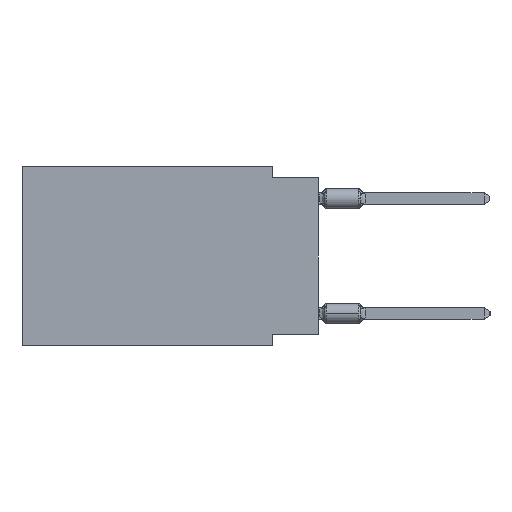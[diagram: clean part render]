
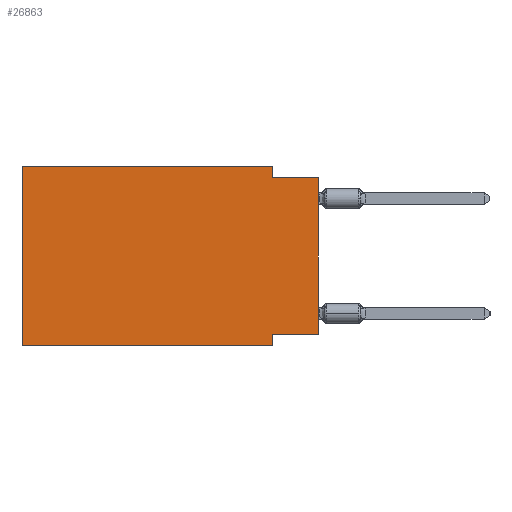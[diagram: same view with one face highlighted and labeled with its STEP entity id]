
A CAD part, left-side view. The second image highlights one B-rep face of the part: STEP entity #26863.
In plain terms, the highlighted planar face has unit normal (-1, 0, 0).
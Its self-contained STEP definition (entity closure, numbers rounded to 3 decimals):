
#726 = DIRECTION ( 'NONE',  ( 1., 0., 0. ) ) ;
#761 = DIRECTION ( 'NONE',  ( 0., -1., 0. ) ) ;
#893 = CARTESIAN_POINT ( 'NONE',  ( 0., 0., -0.635 ) ) ;
#2442 = CARTESIAN_POINT ( 'NONE',  ( 0., 16.383, 0. ) ) ;
#2664 = EDGE_CURVE ( 'NONE', #21408, #15337, #25384, .T. ) ;
#2811 = VECTOR ( 'NONE', #15231, 1000. ) ;
#2906 = CARTESIAN_POINT ( 'NONE',  ( 0., 16.383, 0. ) ) ;
#3596 = CARTESIAN_POINT ( 'NONE',  ( 0., 16.383, 0. ) ) ;
#4561 = CARTESIAN_POINT ( 'NONE',  ( 0., 0., -9.271 ) ) ;
#4688 = EDGE_CURVE ( 'NONE', #7468, #21409, #24923, .T. ) ;
#4941 = LINE ( 'NONE', #11500, #24277 ) ;
#5192 = ORIENTED_EDGE ( 'NONE', *, *, #26535, .F. ) ;
#5665 = DIRECTION ( 'NONE',  ( 0., -1., 0. ) ) ;
#6040 = EDGE_CURVE ( 'NONE', #21409, #11029, #25599, .T. ) ;
#6511 = VECTOR ( 'NONE', #23349, 1000. ) ;
#6889 = CARTESIAN_POINT ( 'NONE',  ( 0., 2.54, -9.906 ) ) ;
#7031 = LINE ( 'NONE', #893, #7467 ) ;
#7324 = CARTESIAN_POINT ( 'NONE',  ( 0., 16.383, -9.906 ) ) ;
#7371 = CARTESIAN_POINT ( 'NONE',  ( 0., 2.54, -0.635 ) ) ;
#7467 = VECTOR ( 'NONE', #761, 1000. ) ;
#7468 = VERTEX_POINT ( 'NONE', #4561 ) ;
#7469 = CARTESIAN_POINT ( 'NONE',  ( 0., 0., 0. ) ) ;
#7603 = LINE ( 'NONE', #7469, #16315 ) ;
#8016 = CARTESIAN_POINT ( 'NONE',  ( 0., 2.54, 0. ) ) ;
#8132 = CARTESIAN_POINT ( 'NONE',  ( 0., 0., -9.271 ) ) ;
#8388 = VECTOR ( 'NONE', #8727, 1000. ) ;
#8727 = DIRECTION ( 'NONE',  ( 0., -1., 0. ) ) ;
#9882 = CARTESIAN_POINT ( 'NONE',  ( 0., 2.54, -9.271 ) ) ;
#11029 = VERTEX_POINT ( 'NONE', #19160 ) ;
#11500 = CARTESIAN_POINT ( 'NONE',  ( 0., 2.54, 0. ) ) ;
#12219 = CARTESIAN_POINT ( 'NONE',  ( 0., 16.383, -9.906 ) ) ;
#13014 = FACE_OUTER_BOUND ( 'NONE', #25684, .T. ) ;
#13268 = CARTESIAN_POINT ( 'NONE',  ( 0., 0., -0.635 ) ) ;
#13796 = ORIENTED_EDGE ( 'NONE', *, *, #2664, .F. ) ;
#14066 = ORIENTED_EDGE ( 'NONE', *, *, #6040, .F. ) ;
#14320 = VERTEX_POINT ( 'NONE', #13268 ) ;
#14914 = VERTEX_POINT ( 'NONE', #7371 ) ;
#15148 = CARTESIAN_POINT ( 'NONE',  ( 0., 16.383, 0. ) ) ;
#15231 = DIRECTION ( 'NONE',  ( 0., 0., -1. ) ) ;
#15337 = VERTEX_POINT ( 'NONE', #8016 ) ;
#15478 = PLANE ( 'NONE',  #26652 ) ;
#15600 = VECTOR ( 'NONE', #5665, 1000. ) ;
#16234 = EDGE_CURVE ( 'NONE', #20782, #21408, #17198, .T. ) ;
#16315 = VECTOR ( 'NONE', #17980, 1000. ) ;
#17198 = LINE ( 'NONE', #15148, #6511 ) ;
#17717 = VECTOR ( 'NONE', #24647, 1000. ) ;
#17980 = DIRECTION ( 'NONE',  ( 0., 0., 1. ) ) ;
#18191 = ORIENTED_EDGE ( 'NONE', *, *, #19741, .T. ) ;
#18731 = EDGE_CURVE ( 'NONE', #15337, #14914, #4941, .T. ) ;
#19160 = CARTESIAN_POINT ( 'NONE',  ( 0., 2.54, -9.906 ) ) ;
#19562 = DIRECTION ( 'NONE',  ( 0., 0., -1. ) ) ;
#19741 = EDGE_CURVE ( 'NONE', #20782, #11029, #22338, .T. ) ;
#20718 = ORIENTED_EDGE ( 'NONE', *, *, #4688, .F. ) ;
#20782 = VERTEX_POINT ( 'NONE', #7324 ) ;
#21408 = VERTEX_POINT ( 'NONE', #3596 ) ;
#21409 = VERTEX_POINT ( 'NONE', #9882 ) ;
#22338 = LINE ( 'NONE', #12219, #15600 ) ;
#23349 = DIRECTION ( 'NONE',  ( 0., 0., 1. ) ) ;
#23938 = EDGE_CURVE ( 'NONE', #7468, #14320, #7603, .T. ) ;
#24277 = VECTOR ( 'NONE', #26215, 1000. ) ;
#24647 = DIRECTION ( 'NONE',  ( 0., 1., 0. ) ) ;
#24878 = ORIENTED_EDGE ( 'NONE', *, *, #23938, .T. ) ;
#24923 = LINE ( 'NONE', #8132, #17717 ) ;
#25384 = LINE ( 'NONE', #2442, #8388 ) ;
#25599 = LINE ( 'NONE', #6889, #2811 ) ;
#25684 = EDGE_LOOP ( 'NONE', ( #24878, #5192, #26216, #13796, #26039, #18191, #14066, #20718 ) ) ;
#26039 = ORIENTED_EDGE ( 'NONE', *, *, #16234, .F. ) ;
#26215 = DIRECTION ( 'NONE',  ( 0., 0., -1. ) ) ;
#26216 = ORIENTED_EDGE ( 'NONE', *, *, #18731, .F. ) ;
#26535 = EDGE_CURVE ( 'NONE', #14914, #14320, #7031, .T. ) ;
#26652 = AXIS2_PLACEMENT_3D ( 'NONE', #2906, #726, #19562 ) ;
#26863 = ADVANCED_FACE ( 'NONE', ( #13014 ), #15478, .F. ) ;
